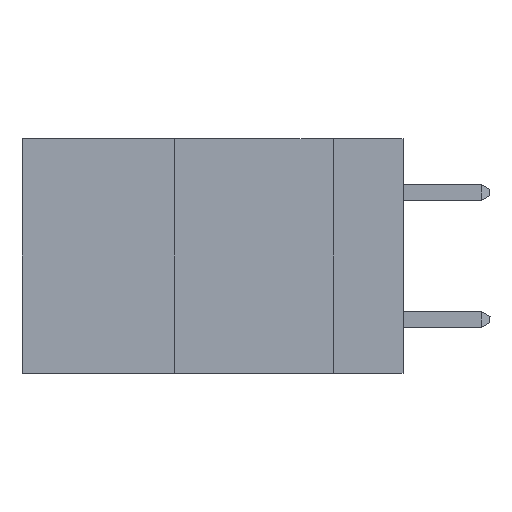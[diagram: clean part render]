
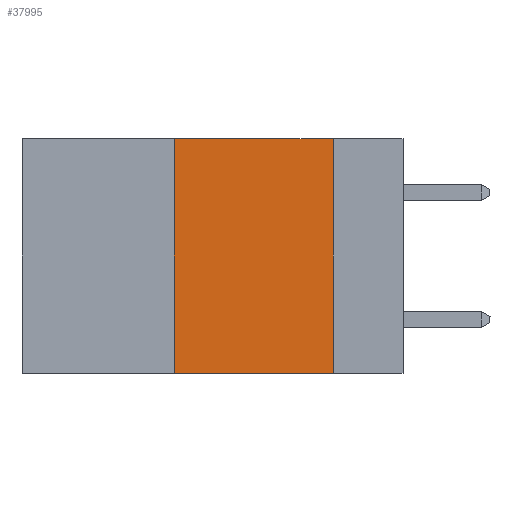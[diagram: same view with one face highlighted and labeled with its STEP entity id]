
A CAD part, left-side view. The second image highlights one B-rep face of the part: STEP entity #37995.
In plain terms, the highlighted planar face has unit normal (-1, 0, 0).
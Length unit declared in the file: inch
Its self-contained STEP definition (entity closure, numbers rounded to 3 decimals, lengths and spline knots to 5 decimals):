
#548 = DIRECTION ( 'NONE',  ( 0., -1., 0. ) ) ;
#813 = CARTESIAN_POINT ( 'NONE',  ( 0., 0.6, 0. ) ) ;
#1703 = FACE_OUTER_BOUND ( 'NONE', #21298, .T. ) ;
#1754 = CARTESIAN_POINT ( 'NONE',  ( 0., 0.11, 0. ) ) ;
#1934 = CARTESIAN_POINT ( 'NONE',  ( 0., 0.36, 0. ) ) ;
#2632 = ORIENTED_EDGE ( 'NONE', *, *, #14649, .F. ) ;
#4331 = LINE ( 'NONE', #27261, #27409 ) ;
#4600 = DIRECTION ( 'NONE',  ( 0., 0., -1. ) ) ;
#7654 = EDGE_CURVE ( 'NONE', #12337, #34484, #10832, .T. ) ;
#10535 = VERTEX_POINT ( 'NONE', #30777 ) ;
#10832 = LINE ( 'NONE', #33705, #34676 ) ;
#11206 = ORIENTED_EDGE ( 'NONE', *, *, #12582, .F. ) ;
#12337 = VERTEX_POINT ( 'NONE', #27170 ) ;
#12582 = EDGE_CURVE ( 'NONE', #10535, #34484, #25774, .T. ) ;
#14649 = EDGE_CURVE ( 'NONE', #15755, #10535, #4331, .T. ) ;
#15755 = VERTEX_POINT ( 'NONE', #1934 ) ;
#16269 = ORIENTED_EDGE ( 'NONE', *, *, #7654, .T. ) ;
#17365 = VECTOR ( 'NONE', #35768, 39.37008 ) ;
#21298 = EDGE_LOOP ( 'NONE', ( #11206, #2632, #23133, #16269 ) ) ;
#23133 = ORIENTED_EDGE ( 'NONE', *, *, #35549, .F. ) ;
#24616 = DIRECTION ( 'NONE',  ( 1., 0., 0. ) ) ;
#25774 = LINE ( 'NONE', #1754, #17365 ) ;
#27170 = CARTESIAN_POINT ( 'NONE',  ( 0., 0.36, -0.37 ) ) ;
#27261 = CARTESIAN_POINT ( 'NONE',  ( 0., 0.6, 0. ) ) ;
#27409 = VECTOR ( 'NONE', #548, 39.37008 ) ;
#30777 = CARTESIAN_POINT ( 'NONE',  ( 0., 0.11, 0. ) ) ;
#31266 = DIRECTION ( 'NONE',  ( 0., -1., 0. ) ) ;
#31297 = PLANE ( 'NONE',  #33624 ) ;
#33624 = AXIS2_PLACEMENT_3D ( 'NONE', #813, #24616, #4600 ) ;
#33705 = CARTESIAN_POINT ( 'NONE',  ( 0., 0.6, -0.37 ) ) ;
#34484 = VERTEX_POINT ( 'NONE', #42287 ) ;
#34676 = VECTOR ( 'NONE', #31266, 39.37008 ) ;
#35549 = EDGE_CURVE ( 'NONE', #12337, #15755, #40316, .T. ) ;
#35768 = DIRECTION ( 'NONE',  ( 0., 0., -1. ) ) ;
#36285 = DIRECTION ( 'NONE',  ( 0., 0., 1. ) ) ;
#36734 = CARTESIAN_POINT ( 'NONE',  ( 0., 0.36, 0. ) ) ;
#37995 = ADVANCED_FACE ( 'NONE', ( #1703 ), #31297, .F. ) ;
#38660 = VECTOR ( 'NONE', #36285, 39.37008 ) ;
#40316 = LINE ( 'NONE', #36734, #38660 ) ;
#42287 = CARTESIAN_POINT ( 'NONE',  ( 0., 0.11, -0.37 ) ) ;
